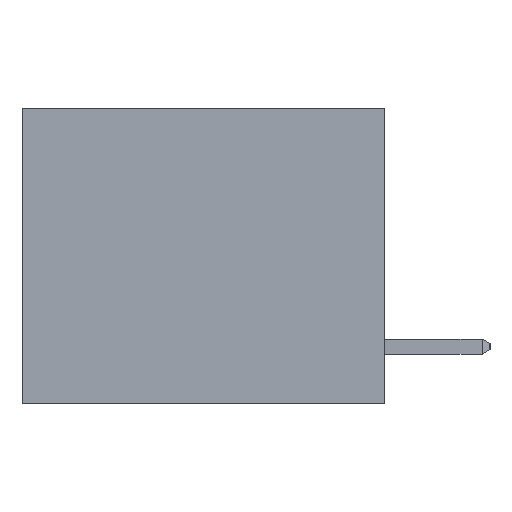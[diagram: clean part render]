
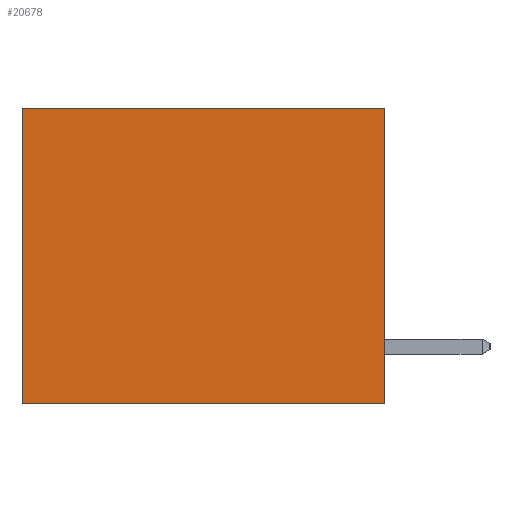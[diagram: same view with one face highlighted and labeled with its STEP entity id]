
A CAD part, left-side view. The second image highlights one B-rep face of the part: STEP entity #20678.
In plain terms, the highlighted planar face has unit normal (-1, 0, 0).
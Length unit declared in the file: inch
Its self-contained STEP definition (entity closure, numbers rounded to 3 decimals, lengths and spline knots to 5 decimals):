
#614 = VERTEX_POINT ( 'NONE', #20544 ) ;
#1312 = DIRECTION ( 'NONE',  ( 1., 0., 0. ) ) ;
#1720 = VERTEX_POINT ( 'NONE', #6493 ) ;
#1783 = AXIS2_PLACEMENT_3D ( 'NONE', #14334, #1312, #5015 ) ;
#1800 = CARTESIAN_POINT ( 'NONE',  ( 0.3165, 0., -0.49 ) ) ;
#1815 = EDGE_CURVE ( 'NONE', #614, #1720, #5671, .T. ) ;
#2115 = CARTESIAN_POINT ( 'NONE',  ( 0.3165, 0., 0. ) ) ;
#4392 = LINE ( 'NONE', #1800, #16893 ) ;
#4852 = EDGE_CURVE ( 'NONE', #18467, #7130, #11501, .T. ) ;
#4991 = ORIENTED_EDGE ( 'NONE', *, *, #1815, .F. ) ;
#5015 = DIRECTION ( 'NONE',  ( 0., 0., -1. ) ) ;
#5561 = CARTESIAN_POINT ( 'NONE',  ( 0.3165, 0.6, 0. ) ) ;
#5671 = LINE ( 'NONE', #11781, #17925 ) ;
#6456 = CARTESIAN_POINT ( 'NONE',  ( 0.3165, 0.6, -0.49 ) ) ;
#6493 = CARTESIAN_POINT ( 'NONE',  ( 0.3165, 0.6, -0.49 ) ) ;
#7130 = VERTEX_POINT ( 'NONE', #5561 ) ;
#8775 = EDGE_LOOP ( 'NONE', ( #17716, #4991, #13932, #17303 ) ) ;
#10745 = EDGE_CURVE ( 'NONE', #18467, #614, #4392, .T. ) ;
#11031 = PLANE ( 'NONE',  #1783 ) ;
#11486 = DIRECTION ( 'NONE',  ( 0., 0., -1. ) ) ;
#11501 = LINE ( 'NONE', #2115, #11757 ) ;
#11656 = DIRECTION ( 'NONE',  ( 0., 0., -1. ) ) ;
#11757 = VECTOR ( 'NONE', #13569, 39.37008 ) ;
#11781 = CARTESIAN_POINT ( 'NONE',  ( 0.3165, 0., -0.49 ) ) ;
#12475 = CARTESIAN_POINT ( 'NONE',  ( 0.3165, 0., 0. ) ) ;
#13019 = LINE ( 'NONE', #6456, #20469 ) ;
#13569 = DIRECTION ( 'NONE',  ( 0., 1., 0. ) ) ;
#13932 = ORIENTED_EDGE ( 'NONE', *, *, #10745, .F. ) ;
#14334 = CARTESIAN_POINT ( 'NONE',  ( 0.3165, 0., -0.49 ) ) ;
#16757 = DIRECTION ( 'NONE',  ( 0., 1., 0. ) ) ;
#16893 = VECTOR ( 'NONE', #11656, 39.37008 ) ;
#17303 = ORIENTED_EDGE ( 'NONE', *, *, #4852, .T. ) ;
#17716 = ORIENTED_EDGE ( 'NONE', *, *, #18231, .T. ) ;
#17925 = VECTOR ( 'NONE', #16757, 39.37008 ) ;
#18231 = EDGE_CURVE ( 'NONE', #7130, #1720, #13019, .T. ) ;
#18467 = VERTEX_POINT ( 'NONE', #12475 ) ;
#19444 = FACE_OUTER_BOUND ( 'NONE', #8775, .T. ) ;
#20469 = VECTOR ( 'NONE', #11486, 39.37008 ) ;
#20544 = CARTESIAN_POINT ( 'NONE',  ( 0.3165, 0., -0.49 ) ) ;
#20678 = ADVANCED_FACE ( 'NONE', ( #19444 ), #11031, .F. ) ;
